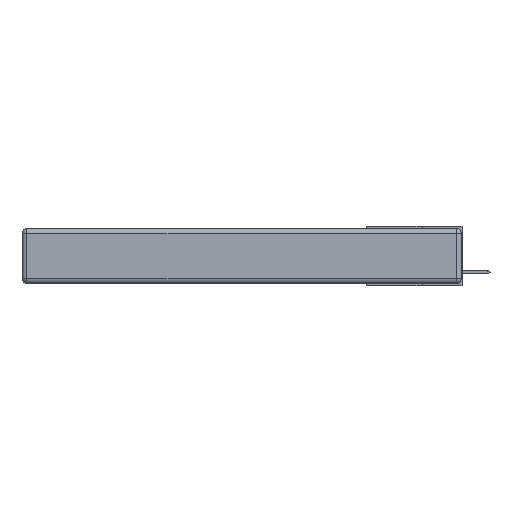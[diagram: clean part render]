
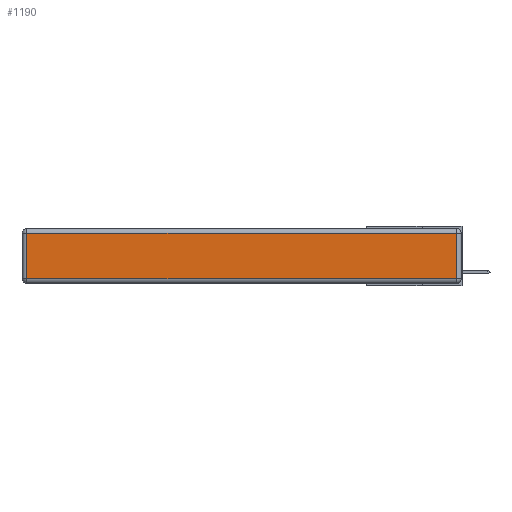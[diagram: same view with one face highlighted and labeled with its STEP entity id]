
A CAD part, left-side view. The second image highlights one B-rep face of the part: STEP entity #1190.
In plain terms, the highlighted planar face has unit normal (-1, 0, 0).
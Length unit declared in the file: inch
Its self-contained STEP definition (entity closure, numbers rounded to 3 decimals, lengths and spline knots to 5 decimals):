
#411 = LINE ( 'NONE', #5681, #8587 ) ;
#691 = VECTOR ( 'NONE', #4161, 39.37008 ) ;
#976 = EDGE_CURVE ( 'NONE', #2734, #10343, #4830, .T. ) ;
#1173 = AXIS2_PLACEMENT_3D ( 'NONE', #10974, #2441, #1414 ) ;
#1190 = ADVANCED_FACE ( 'NONE', ( #8316 ), #6844, .T. ) ;
#1261 = DIRECTION ( 'NONE',  ( 0., 1., 0. ) ) ;
#1414 = DIRECTION ( 'NONE',  ( 0., 0., 1. ) ) ;
#1955 = VERTEX_POINT ( 'NONE', #4843 ) ;
#2441 = DIRECTION ( 'NONE',  ( -1., 0., 0. ) ) ;
#2472 = LINE ( 'NONE', #7867, #9153 ) ;
#2733 = VERTEX_POINT ( 'NONE', #11016 ) ;
#2734 = VERTEX_POINT ( 'NONE', #8975 ) ;
#2829 = EDGE_CURVE ( 'NONE', #1955, #2733, #2472, .T. ) ;
#4161 = DIRECTION ( 'NONE',  ( 0., -1., 0. ) ) ;
#4207 = ORIENTED_EDGE ( 'NONE', *, *, #7317, .T. ) ;
#4517 = ORIENTED_EDGE ( 'NONE', *, *, #6299, .T. ) ;
#4830 = LINE ( 'NONE', #7269, #5834 ) ;
#4843 = CARTESIAN_POINT ( 'NONE',  ( 0., 0.03, -0.313 ) ) ;
#5071 = EDGE_LOOP ( 'NONE', ( #4207, #10362, #4517, #6554 ) ) ;
#5309 = CARTESIAN_POINT ( 'NONE',  ( 0., 2.72, -0.313 ) ) ;
#5681 = CARTESIAN_POINT ( 'NONE',  ( 0., 2.75, -0.03 ) ) ;
#5834 = VECTOR ( 'NONE', #11671, 39.37008 ) ;
#6299 = EDGE_CURVE ( 'NONE', #2733, #2734, #411, .T. ) ;
#6554 = ORIENTED_EDGE ( 'NONE', *, *, #976, .T. ) ;
#6844 = PLANE ( 'NONE',  #1173 ) ;
#7269 = CARTESIAN_POINT ( 'NONE',  ( 0., 2.72, -0.343 ) ) ;
#7317 = EDGE_CURVE ( 'NONE', #10343, #1955, #7713, .T. ) ;
#7713 = LINE ( 'NONE', #9420, #691 ) ;
#7867 = CARTESIAN_POINT ( 'NONE',  ( 0., 0.03, -0.343 ) ) ;
#8316 = FACE_OUTER_BOUND ( 'NONE', #5071, .T. ) ;
#8587 = VECTOR ( 'NONE', #1261, 39.37008 ) ;
#8975 = CARTESIAN_POINT ( 'NONE',  ( 0., 2.72, -0.03 ) ) ;
#9153 = VECTOR ( 'NONE', #11157, 39.37008 ) ;
#9420 = CARTESIAN_POINT ( 'NONE',  ( 0., 0., -0.313 ) ) ;
#10343 = VERTEX_POINT ( 'NONE', #5309 ) ;
#10362 = ORIENTED_EDGE ( 'NONE', *, *, #2829, .T. ) ;
#10974 = CARTESIAN_POINT ( 'NONE',  ( 0., 0., -0.343 ) ) ;
#11016 = CARTESIAN_POINT ( 'NONE',  ( 0., 0.03, -0.03 ) ) ;
#11157 = DIRECTION ( 'NONE',  ( 0., 0., 1. ) ) ;
#11671 = DIRECTION ( 'NONE',  ( 0., 0., -1. ) ) ;
